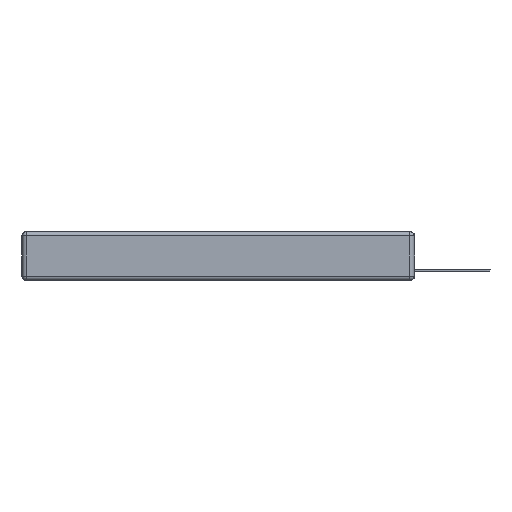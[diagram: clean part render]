
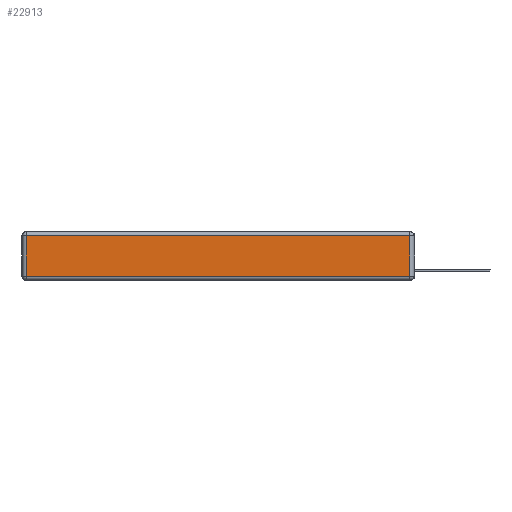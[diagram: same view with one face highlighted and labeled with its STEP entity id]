
A CAD part, left-side view. The second image highlights one B-rep face of the part: STEP entity #22913.
In plain terms, the highlighted planar face has unit normal (-1, 0, 0).
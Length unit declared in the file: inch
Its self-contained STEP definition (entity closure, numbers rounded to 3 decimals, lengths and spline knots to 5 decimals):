
#23 = CARTESIAN_POINT ( 'NONE',  ( 0., 0.03, -0.03 ) ) ;
#28 = EDGE_LOOP ( 'NONE', ( #16402, #13039, #15977, #2531 ) ) ;
#741 = VERTEX_POINT ( 'NONE', #14276 ) ;
#2372 = EDGE_CURVE ( 'NONE', #13438, #19680, #14148, .T. ) ;
#2440 = EDGE_CURVE ( 'NONE', #19680, #4996, #16146, .T. ) ;
#2527 = PLANE ( 'NONE',  #19759 ) ;
#2531 = ORIENTED_EDGE ( 'NONE', *, *, #13498, .T. ) ;
#3772 = CARTESIAN_POINT ( 'NONE',  ( 0., 0., -0.313 ) ) ;
#4791 = VECTOR ( 'NONE', #6041, 39.37008 ) ;
#4996 = VERTEX_POINT ( 'NONE', #23 ) ;
#6041 = DIRECTION ( 'NONE',  ( 0., 0., -1. ) ) ;
#6965 = LINE ( 'NONE', #14145, #21353 ) ;
#6969 = DIRECTION ( 'NONE',  ( 0., -1., 0. ) ) ;
#7827 = LINE ( 'NONE', #14985, #4791 ) ;
#9718 = DIRECTION ( 'NONE',  ( 0., 0., 1. ) ) ;
#11269 = VECTOR ( 'NONE', #6969, 39.37008 ) ;
#12493 = DIRECTION ( 'NONE',  ( 0., 0., 1. ) ) ;
#12702 = CARTESIAN_POINT ( 'NONE',  ( 0., 0.03, -0.313 ) ) ;
#13039 = ORIENTED_EDGE ( 'NONE', *, *, #2440, .T. ) ;
#13438 = VERTEX_POINT ( 'NONE', #18423 ) ;
#13498 = EDGE_CURVE ( 'NONE', #741, #13438, #7827, .T. ) ;
#13811 = EDGE_CURVE ( 'NONE', #4996, #741, #6965, .T. ) ;
#14145 = CARTESIAN_POINT ( 'NONE',  ( 0., 2.75, -0.03 ) ) ;
#14148 = LINE ( 'NONE', #3772, #11269 ) ;
#14276 = CARTESIAN_POINT ( 'NONE',  ( 0., 2.72, -0.03 ) ) ;
#14985 = CARTESIAN_POINT ( 'NONE',  ( 0., 2.72, -0.343 ) ) ;
#15977 = ORIENTED_EDGE ( 'NONE', *, *, #13811, .T. ) ;
#16146 = LINE ( 'NONE', #23130, #21436 ) ;
#16402 = ORIENTED_EDGE ( 'NONE', *, *, #2372, .T. ) ;
#18423 = CARTESIAN_POINT ( 'NONE',  ( 0., 2.72, -0.313 ) ) ;
#18798 = DIRECTION ( 'NONE',  ( -1., 0., 0. ) ) ;
#18832 = DIRECTION ( 'NONE',  ( 0., 1., 0. ) ) ;
#19680 = VERTEX_POINT ( 'NONE', #12702 ) ;
#19759 = AXIS2_PLACEMENT_3D ( 'NONE', #21875, #18798, #9718 ) ;
#21353 = VECTOR ( 'NONE', #18832, 39.37008 ) ;
#21436 = VECTOR ( 'NONE', #12493, 39.37008 ) ;
#21875 = CARTESIAN_POINT ( 'NONE',  ( 0., 0., -0.343 ) ) ;
#22113 = FACE_OUTER_BOUND ( 'NONE', #28, .T. ) ;
#22913 = ADVANCED_FACE ( 'NONE', ( #22113 ), #2527, .T. ) ;
#23130 = CARTESIAN_POINT ( 'NONE',  ( 0., 0.03, -0.343 ) ) ;
